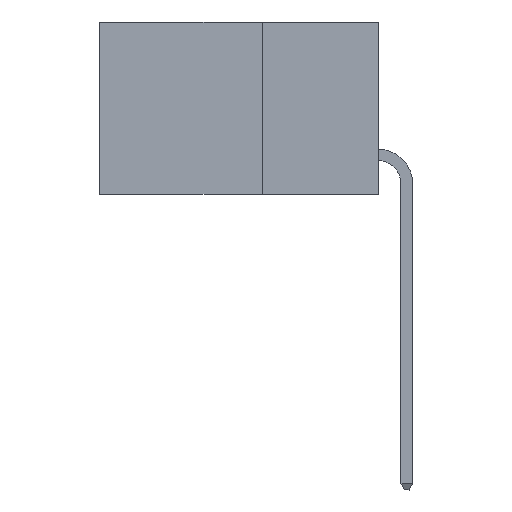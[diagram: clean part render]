
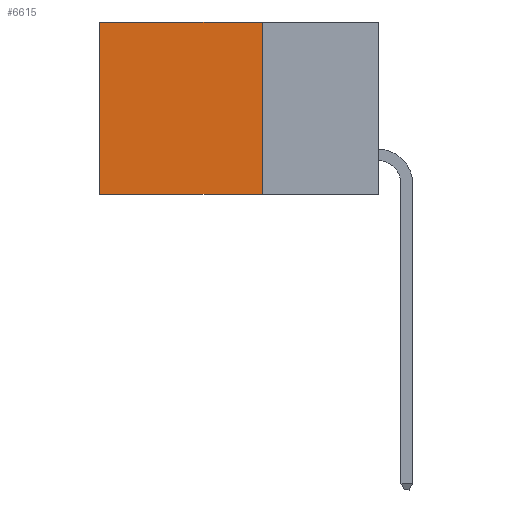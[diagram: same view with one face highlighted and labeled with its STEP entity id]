
A CAD part, left-side view. The second image highlights one B-rep face of the part: STEP entity #6615.
In plain terms, the highlighted planar face has unit normal (-1, 0, 0).
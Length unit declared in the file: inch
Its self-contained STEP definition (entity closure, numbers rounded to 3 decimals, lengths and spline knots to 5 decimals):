
#75 = ORIENTED_EDGE ( 'NONE', *, *, #12502, .F. ) ;
#594 = CARTESIAN_POINT ( 'NONE',  ( 0.2615, 0.6, 0. ) ) ;
#734 = VECTOR ( 'NONE', #16419, 39.37008 ) ;
#991 = VERTEX_POINT ( 'NONE', #7090 ) ;
#1757 = VERTEX_POINT ( 'NONE', #11152 ) ;
#2587 = VECTOR ( 'NONE', #14889, 39.37008 ) ;
#3230 = DIRECTION ( 'NONE',  ( 1., 0., 0. ) ) ;
#4636 = DIRECTION ( 'NONE',  ( 0., 0., -1. ) ) ;
#4670 = CARTESIAN_POINT ( 'NONE',  ( 0.2615, 0.25, 0. ) ) ;
#4869 = CARTESIAN_POINT ( 'NONE',  ( 0.2615, 0.25, -0.37 ) ) ;
#6058 = ORIENTED_EDGE ( 'NONE', *, *, #6334, .F. ) ;
#6111 = ORIENTED_EDGE ( 'NONE', *, *, #11824, .T. ) ;
#6334 = EDGE_CURVE ( 'NONE', #1757, #13349, #16317, .T. ) ;
#6354 = LINE ( 'NONE', #4670, #2587 ) ;
#6615 = ADVANCED_FACE ( 'NONE', ( #13158 ), #16273, .F. ) ;
#6881 = LINE ( 'NONE', #8377, #8942 ) ;
#7090 = CARTESIAN_POINT ( 'NONE',  ( 0.2615, 0.6, -0.37 ) ) ;
#8341 = DIRECTION ( 'NONE',  ( 0., 1., 0. ) ) ;
#8377 = CARTESIAN_POINT ( 'NONE',  ( 0.2615, 0.6, -0.37 ) ) ;
#8441 = CARTESIAN_POINT ( 'NONE',  ( 0.2615, 0.25, -0.37 ) ) ;
#8912 = CARTESIAN_POINT ( 'NONE',  ( 0.2615, 0.25, -0.37 ) ) ;
#8942 = VECTOR ( 'NONE', #20192, 39.37008 ) ;
#9015 = EDGE_CURVE ( 'NONE', #11996, #991, #6881, .T. ) ;
#9748 = VECTOR ( 'NONE', #8341, 39.37008 ) ;
#11152 = CARTESIAN_POINT ( 'NONE',  ( 0.2615, 0.25, 0. ) ) ;
#11619 = EDGE_LOOP ( 'NONE', ( #17208, #75, #6058, #6111 ) ) ;
#11824 = EDGE_CURVE ( 'NONE', #1757, #11996, #6354, .T. ) ;
#11996 = VERTEX_POINT ( 'NONE', #594 ) ;
#12502 = EDGE_CURVE ( 'NONE', #13349, #991, #15082, .T. ) ;
#13158 = FACE_OUTER_BOUND ( 'NONE', #11619, .T. ) ;
#13349 = VERTEX_POINT ( 'NONE', #8912 ) ;
#14074 = AXIS2_PLACEMENT_3D ( 'NONE', #14568, #3230, #4636 ) ;
#14568 = CARTESIAN_POINT ( 'NONE',  ( 0.2615, 0.25, -0.37 ) ) ;
#14889 = DIRECTION ( 'NONE',  ( 0., 1., 0. ) ) ;
#15082 = LINE ( 'NONE', #8441, #9748 ) ;
#16273 = PLANE ( 'NONE',  #14074 ) ;
#16317 = LINE ( 'NONE', #4869, #734 ) ;
#16419 = DIRECTION ( 'NONE',  ( 0., 0., -1. ) ) ;
#17208 = ORIENTED_EDGE ( 'NONE', *, *, #9015, .T. ) ;
#20192 = DIRECTION ( 'NONE',  ( 0., 0., -1. ) ) ;
